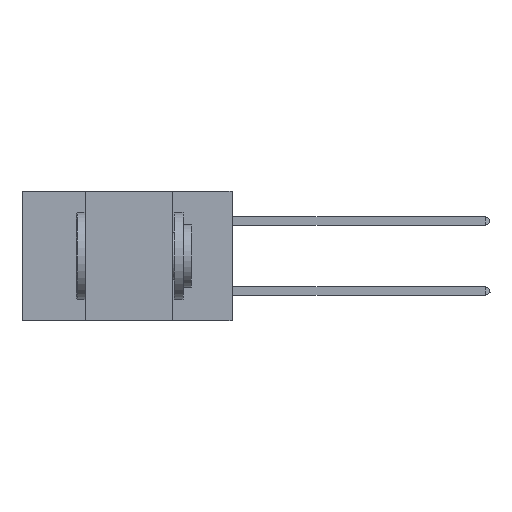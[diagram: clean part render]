
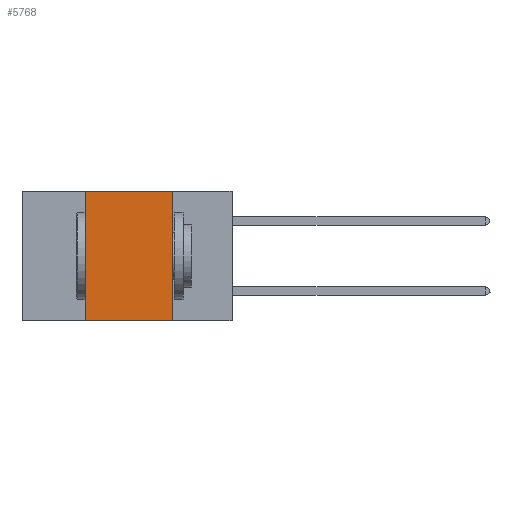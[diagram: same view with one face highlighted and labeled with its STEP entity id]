
A CAD part, left-side view. The second image highlights one B-rep face of the part: STEP entity #5768.
In plain terms, the highlighted planar face has unit normal (-1, 0, 0).
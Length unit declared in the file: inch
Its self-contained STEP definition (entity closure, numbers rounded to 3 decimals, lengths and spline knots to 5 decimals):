
#992 = CARTESIAN_POINT ( 'NONE',  ( 0., 0.42, -0.37 ) ) ;
#1187 = EDGE_CURVE ( 'NONE', #16992, #2179, #18484, .T. ) ;
#2179 = VERTEX_POINT ( 'NONE', #16185 ) ;
#3304 = VECTOR ( 'NONE', #25821, 39.37008 ) ;
#3405 = CARTESIAN_POINT ( 'NONE',  ( 0., 0.6, 0. ) ) ;
#3865 = LINE ( 'NONE', #19796, #31194 ) ;
#4738 = AXIS2_PLACEMENT_3D ( 'NONE', #23934, #32808, #33050 ) ;
#5768 = ADVANCED_FACE ( 'NONE', ( #12815 ), #24059, .F. ) ;
#8098 = LINE ( 'NONE', #9051, #18868 ) ;
#9051 = CARTESIAN_POINT ( 'NONE',  ( 0., 0.6, -0.37 ) ) ;
#12815 = FACE_OUTER_BOUND ( 'NONE', #34434, .T. ) ;
#16185 = CARTESIAN_POINT ( 'NONE',  ( 0., 0.17, 0. ) ) ;
#16992 = VERTEX_POINT ( 'NONE', #17961 ) ;
#17030 = EDGE_CURVE ( 'NONE', #31136, #29609, #8098, .T. ) ;
#17961 = CARTESIAN_POINT ( 'NONE',  ( 0., 0.42, 0. ) ) ;
#18484 = LINE ( 'NONE', #3405, #19386 ) ;
#18868 = VECTOR ( 'NONE', #20572, 39.37008 ) ;
#19386 = VECTOR ( 'NONE', #35048, 39.37008 ) ;
#19515 = EDGE_CURVE ( 'NONE', #2179, #29609, #27029, .T. ) ;
#19796 = CARTESIAN_POINT ( 'NONE',  ( 0., 0.42, 0. ) ) ;
#19935 = ORIENTED_EDGE ( 'NONE', *, *, #35952, .F. ) ;
#20484 = CARTESIAN_POINT ( 'NONE',  ( 0., 0.17, 0. ) ) ;
#20572 = DIRECTION ( 'NONE',  ( 0., -1., 0. ) ) ;
#23334 = ORIENTED_EDGE ( 'NONE', *, *, #1187, .F. ) ;
#23934 = CARTESIAN_POINT ( 'NONE',  ( 0., 0.6, 0. ) ) ;
#24059 = PLANE ( 'NONE',  #4738 ) ;
#25821 = DIRECTION ( 'NONE',  ( 0., 0., -1. ) ) ;
#27029 = LINE ( 'NONE', #20484, #3304 ) ;
#29609 = VERTEX_POINT ( 'NONE', #31781 ) ;
#30626 = DIRECTION ( 'NONE',  ( 0., 0., 1. ) ) ;
#31136 = VERTEX_POINT ( 'NONE', #992 ) ;
#31194 = VECTOR ( 'NONE', #30626, 39.37008 ) ;
#31781 = CARTESIAN_POINT ( 'NONE',  ( 0., 0.17, -0.37 ) ) ;
#32808 = DIRECTION ( 'NONE',  ( 1., 0., 0. ) ) ;
#33019 = ORIENTED_EDGE ( 'NONE', *, *, #19515, .F. ) ;
#33050 = DIRECTION ( 'NONE',  ( 0., 0., -1. ) ) ;
#34434 = EDGE_LOOP ( 'NONE', ( #33019, #23334, #19935, #34532 ) ) ;
#34532 = ORIENTED_EDGE ( 'NONE', *, *, #17030, .T. ) ;
#35048 = DIRECTION ( 'NONE',  ( 0., -1., 0. ) ) ;
#35952 = EDGE_CURVE ( 'NONE', #31136, #16992, #3865, .T. ) ;
